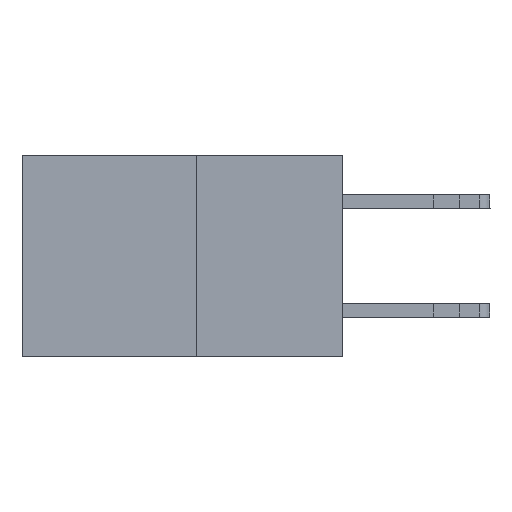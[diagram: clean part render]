
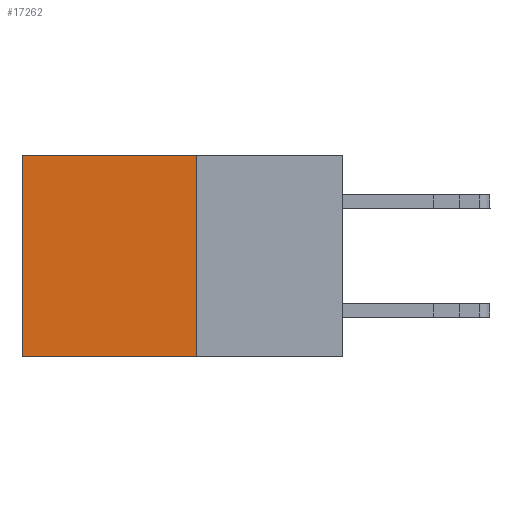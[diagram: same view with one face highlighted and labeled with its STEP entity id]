
A CAD part, left-side view. The second image highlights one B-rep face of the part: STEP entity #17262.
In plain terms, the highlighted planar face has unit normal (-1, 0, 0).
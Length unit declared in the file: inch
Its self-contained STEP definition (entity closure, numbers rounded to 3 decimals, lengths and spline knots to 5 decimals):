
#314 = PLANE ( 'NONE',  #5766 ) ;
#1579 = CARTESIAN_POINT ( 'NONE',  ( 0.277, 0.59, -0.37 ) ) ;
#1596 = VERTEX_POINT ( 'NONE', #7036 ) ;
#1829 = DIRECTION ( 'NONE',  ( 0., 0., -1. ) ) ;
#1934 = CARTESIAN_POINT ( 'NONE',  ( 0.277, 0.59, -0.37 ) ) ;
#2630 = VECTOR ( 'NONE', #9142, 39.37008 ) ;
#3419 = CARTESIAN_POINT ( 'NONE',  ( 0.277, 0.27, 0. ) ) ;
#3780 = VERTEX_POINT ( 'NONE', #3419 ) ;
#3939 = VERTEX_POINT ( 'NONE', #1934 ) ;
#4396 = CARTESIAN_POINT ( 'NONE',  ( 0.277, 0.27, 0. ) ) ;
#4569 = LINE ( 'NONE', #13615, #8537 ) ;
#5607 = ORIENTED_EDGE ( 'NONE', *, *, #8465, .T. ) ;
#5766 = AXIS2_PLACEMENT_3D ( 'NONE', #9370, #10867, #1829 ) ;
#5863 = EDGE_CURVE ( 'NONE', #3780, #6250, #4569, .T. ) ;
#6250 = VERTEX_POINT ( 'NONE', #14141 ) ;
#6297 = VECTOR ( 'NONE', #11493, 39.37008 ) ;
#7036 = CARTESIAN_POINT ( 'NONE',  ( 0.277, 0.59, 0. ) ) ;
#8442 = CARTESIAN_POINT ( 'NONE',  ( 0.277, 0.27, -0.37 ) ) ;
#8465 = EDGE_CURVE ( 'NONE', #3780, #1596, #15250, .T. ) ;
#8537 = VECTOR ( 'NONE', #13852, 39.37008 ) ;
#9142 = DIRECTION ( 'NONE',  ( 0., 0., -1. ) ) ;
#9370 = CARTESIAN_POINT ( 'NONE',  ( 0.277, 0.27, -0.37 ) ) ;
#10193 = FACE_OUTER_BOUND ( 'NONE', #13256, .T. ) ;
#10318 = EDGE_CURVE ( 'NONE', #6250, #3939, #13808, .T. ) ;
#10867 = DIRECTION ( 'NONE',  ( 1., 0., 0. ) ) ;
#11493 = DIRECTION ( 'NONE',  ( 0., 1., 0. ) ) ;
#12660 = ORIENTED_EDGE ( 'NONE', *, *, #13732, .T. ) ;
#13256 = EDGE_LOOP ( 'NONE', ( #12660, #13805, #18105, #5607 ) ) ;
#13462 = DIRECTION ( 'NONE',  ( 0., 1., 0. ) ) ;
#13615 = CARTESIAN_POINT ( 'NONE',  ( 0.277, 0.27, -0.37 ) ) ;
#13732 = EDGE_CURVE ( 'NONE', #1596, #3939, #18443, .T. ) ;
#13805 = ORIENTED_EDGE ( 'NONE', *, *, #10318, .F. ) ;
#13808 = LINE ( 'NONE', #8442, #6297 ) ;
#13852 = DIRECTION ( 'NONE',  ( 0., 0., -1. ) ) ;
#14141 = CARTESIAN_POINT ( 'NONE',  ( 0.277, 0.27, -0.37 ) ) ;
#14341 = VECTOR ( 'NONE', #13462, 39.37008 ) ;
#15250 = LINE ( 'NONE', #4396, #14341 ) ;
#17262 = ADVANCED_FACE ( 'NONE', ( #10193 ), #314, .F. ) ;
#18105 = ORIENTED_EDGE ( 'NONE', *, *, #5863, .F. ) ;
#18443 = LINE ( 'NONE', #1579, #2630 ) ;
